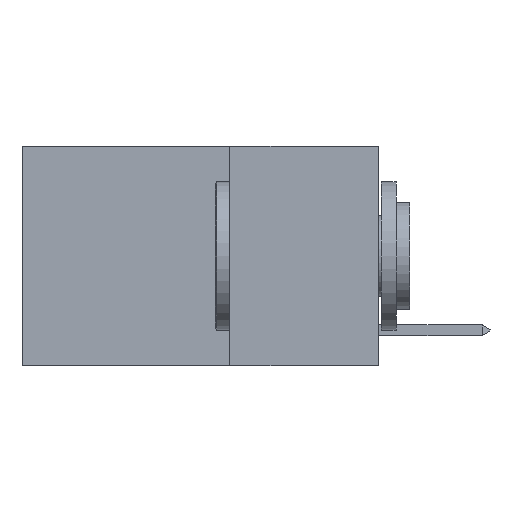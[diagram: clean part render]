
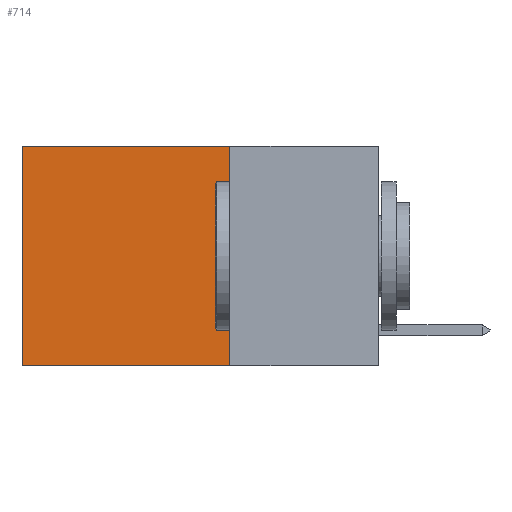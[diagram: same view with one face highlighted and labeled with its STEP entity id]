
A CAD part, left-side view. The second image highlights one B-rep face of the part: STEP entity #714.
In plain terms, the highlighted planar face has unit normal (-1, 0, 0).
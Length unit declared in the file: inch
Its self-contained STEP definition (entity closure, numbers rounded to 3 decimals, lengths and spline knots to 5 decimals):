
#635 = CARTESIAN_POINT ( 'NONE',  ( 0.2625, 0.6, 0. ) ) ;
#714 = ADVANCED_FACE ( 'NONE', ( #25566 ), #15769, .F. ) ;
#2702 = VECTOR ( 'NONE', #9277, 39.37008 ) ;
#3036 = CARTESIAN_POINT ( 'NONE',  ( 0.2625, 0.25, 0. ) ) ;
#3839 = VERTEX_POINT ( 'NONE', #22215 ) ;
#4624 = CARTESIAN_POINT ( 'NONE',  ( 0.2625, 0.25, 0. ) ) ;
#5071 = CARTESIAN_POINT ( 'NONE',  ( 0.2625, 0.6, 0. ) ) ;
#6276 = EDGE_CURVE ( 'NONE', #21033, #3839, #21464, .T. ) ;
#7991 = ORIENTED_EDGE ( 'NONE', *, *, #13709, .F. ) ;
#8564 = ORIENTED_EDGE ( 'NONE', *, *, #6276, .T. ) ;
#9277 = DIRECTION ( 'NONE',  ( 0., 1., 0. ) ) ;
#9438 = EDGE_CURVE ( 'NONE', #24643, #21033, #13613, .T. ) ;
#9915 = VECTOR ( 'NONE', #24933, 39.37008 ) ;
#10610 = CARTESIAN_POINT ( 'NONE',  ( 0.2625, 0.25, -0.37 ) ) ;
#10721 = VECTOR ( 'NONE', #12651, 39.37008 ) ;
#12651 = DIRECTION ( 'NONE',  ( 0., 1., 0. ) ) ;
#13150 = ORIENTED_EDGE ( 'NONE', *, *, #9438, .T. ) ;
#13613 = LINE ( 'NONE', #3036, #2702 ) ;
#13709 = EDGE_CURVE ( 'NONE', #24643, #21209, #20078, .T. ) ;
#14927 = DIRECTION ( 'NONE',  ( 0., 0., -1. ) ) ;
#14953 = DIRECTION ( 'NONE',  ( 1., 0., 0. ) ) ;
#15041 = CARTESIAN_POINT ( 'NONE',  ( 0.2625, 0.25, 0. ) ) ;
#15712 = CARTESIAN_POINT ( 'NONE',  ( 0.2625, 0.25, 0. ) ) ;
#15769 = PLANE ( 'NONE',  #25718 ) ;
#16750 = LINE ( 'NONE', #10610, #10721 ) ;
#19101 = DIRECTION ( 'NONE',  ( 0., 0., -1. ) ) ;
#20078 = LINE ( 'NONE', #4624, #9915 ) ;
#21033 = VERTEX_POINT ( 'NONE', #5071 ) ;
#21209 = VERTEX_POINT ( 'NONE', #25885 ) ;
#21464 = LINE ( 'NONE', #635, #25466 ) ;
#22215 = CARTESIAN_POINT ( 'NONE',  ( 0.2625, 0.6, -0.37 ) ) ;
#23894 = EDGE_LOOP ( 'NONE', ( #8564, #24470, #7991, #13150 ) ) ;
#24470 = ORIENTED_EDGE ( 'NONE', *, *, #24913, .F. ) ;
#24643 = VERTEX_POINT ( 'NONE', #15041 ) ;
#24913 = EDGE_CURVE ( 'NONE', #21209, #3839, #16750, .T. ) ;
#24933 = DIRECTION ( 'NONE',  ( 0., 0., -1. ) ) ;
#25466 = VECTOR ( 'NONE', #19101, 39.37008 ) ;
#25566 = FACE_OUTER_BOUND ( 'NONE', #23894, .T. ) ;
#25718 = AXIS2_PLACEMENT_3D ( 'NONE', #15712, #14953, #14927 ) ;
#25885 = CARTESIAN_POINT ( 'NONE',  ( 0.2625, 0.25, -0.37 ) ) ;
